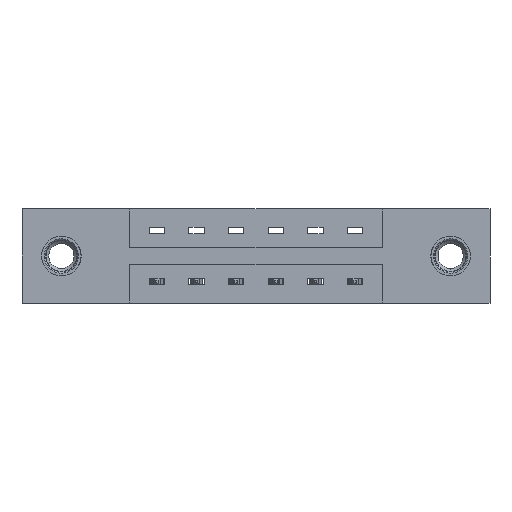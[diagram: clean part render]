
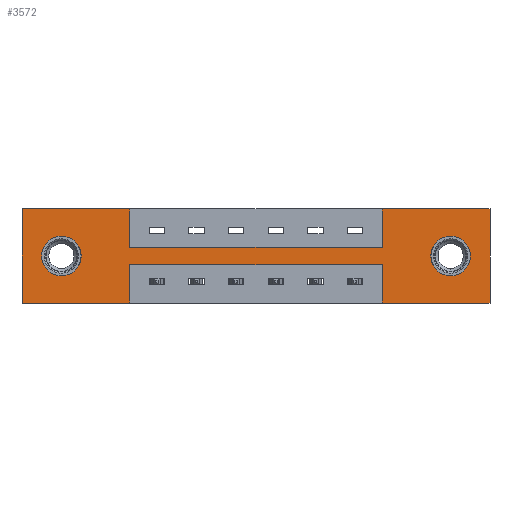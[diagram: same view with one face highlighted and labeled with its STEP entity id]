
A CAD part, front view. The second image highlights one B-rep face of the part: STEP entity #3572.
In plain terms, the highlighted planar face has unit normal (0, -1, 0).
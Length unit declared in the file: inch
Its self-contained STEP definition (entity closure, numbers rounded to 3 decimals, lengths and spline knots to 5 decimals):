
#15 = ORIENTED_EDGE ( 'NONE', *, *, #8971, .F. ) ;
#354 = LINE ( 'NONE', #3860, #2844 ) ;
#487 = VERTEX_POINT ( 'NONE', #9995 ) ;
#631 = EDGE_CURVE ( 'NONE', #6717, #3321, #6698, .T. ) ;
#673 = FACE_OUTER_BOUND ( 'NONE', #7245, .T. ) ;
#692 = LINE ( 'NONE', #9486, #9682 ) ;
#1028 = DIRECTION ( 'NONE',  ( 0., 0., -1. ) ) ;
#1061 = DIRECTION ( 'NONE',  ( 0., 1., 0. ) ) ;
#1080 = ORIENTED_EDGE ( 'NONE', *, *, #5668, .T. ) ;
#1142 = AXIS2_PLACEMENT_3D ( 'NONE', #9271, #4467, #6088 ) ;
#1146 = DIRECTION ( 'NONE',  ( 0., 0., 1. ) ) ;
#1313 = VECTOR ( 'NONE', #6585, 39.37008 ) ;
#1339 = CARTESIAN_POINT ( 'NONE',  ( 1.842, 0., -0.37 ) ) ;
#1387 = CARTESIAN_POINT ( 'NONE',  ( 0., 0., 0. ) ) ;
#1512 = VERTEX_POINT ( 'NONE', #10016 ) ;
#1695 = DIRECTION ( 'NONE',  ( -1., 0., 0. ) ) ;
#1712 = CARTESIAN_POINT ( 'NONE',  ( 1.842, 0., 0. ) ) ;
#1737 = CARTESIAN_POINT ( 'NONE',  ( 0.425, 0., -0.15 ) ) ;
#1751 = EDGE_CURVE ( 'NONE', #487, #3925, #10070, .T. ) ;
#1791 = VERTEX_POINT ( 'NONE', #8266 ) ;
#1977 = VERTEX_POINT ( 'NONE', #8176 ) ;
#1978 = EDGE_CURVE ( 'NONE', #3321, #1791, #3049, .T. ) ;
#2050 = EDGE_CURVE ( 'NONE', #9061, #5885, #9435, .T. ) ;
#2147 = AXIS2_PLACEMENT_3D ( 'NONE', #2590, #6578, #1028 ) ;
#2290 = DIRECTION ( 'NONE',  ( -1., 0., 0. ) ) ;
#2469 = EDGE_LOOP ( 'NONE', ( #5500, #4221 ) ) ;
#2579 = VERTEX_POINT ( 'NONE', #8426 ) ;
#2590 = CARTESIAN_POINT ( 'NONE',  ( 0., 0., -0.37 ) ) ;
#2623 = PLANE ( 'NONE',  #2147 ) ;
#2844 = VECTOR ( 'NONE', #2290, 39.37008 ) ;
#2908 = EDGE_CURVE ( 'NONE', #6254, #3053, #6924, .T. ) ;
#2949 = EDGE_CURVE ( 'NONE', #5885, #9061, #5907, .T. ) ;
#3049 = LINE ( 'NONE', #8140, #10303 ) ;
#3053 = VERTEX_POINT ( 'NONE', #1339 ) ;
#3117 = ORIENTED_EDGE ( 'NONE', *, *, #9688, .F. ) ;
#3219 = DIRECTION ( 'NONE',  ( 1., 0., 0. ) ) ;
#3321 = VERTEX_POINT ( 'NONE', #5565 ) ;
#3382 = CARTESIAN_POINT ( 'NONE',  ( 0.425, 0., -0.37 ) ) ;
#3572 = ADVANCED_FACE ( 'NONE', ( #8411, #6151, #673 ), #2623, .T. ) ;
#3645 = LINE ( 'NONE', #1737, #8407 ) ;
#3860 = CARTESIAN_POINT ( 'NONE',  ( 0.425, 0., -0.22 ) ) ;
#3925 = VERTEX_POINT ( 'NONE', #4367 ) ;
#3964 = LINE ( 'NONE', #4913, #5933 ) ;
#4069 = VERTEX_POINT ( 'NONE', #9632 ) ;
#4138 = CARTESIAN_POINT ( 'NONE',  ( 0., 0., -0.37 ) ) ;
#4189 = CIRCLE ( 'NONE', #4263, 0.078 ) ;
#4221 = ORIENTED_EDGE ( 'NONE', *, *, #2949, .T. ) ;
#4254 = DIRECTION ( 'NONE',  ( 0., 1., 0. ) ) ;
#4263 = AXIS2_PLACEMENT_3D ( 'NONE', #9015, #4254, #5082 ) ;
#4367 = CARTESIAN_POINT ( 'NONE',  ( 0.425, 0., -0.37 ) ) ;
#4467 = DIRECTION ( 'NONE',  ( 0., 1., 0. ) ) ;
#4578 = VECTOR ( 'NONE', #8750, 39.37008 ) ;
#4743 = EDGE_CURVE ( 'NONE', #7360, #487, #354, .T. ) ;
#4784 = VECTOR ( 'NONE', #7283, 39.37008 ) ;
#4875 = ORIENTED_EDGE ( 'NONE', *, *, #1751, .F. ) ;
#4887 = EDGE_CURVE ( 'NONE', #1512, #7360, #3964, .T. ) ;
#4913 = CARTESIAN_POINT ( 'NONE',  ( 1.417, 0., -0.37 ) ) ;
#4977 = DIRECTION ( 'NONE',  ( 0., 0., 1. ) ) ;
#5082 = DIRECTION ( 'NONE',  ( 0., 0., -1. ) ) ;
#5191 = ORIENTED_EDGE ( 'NONE', *, *, #631, .F. ) ;
#5242 = CARTESIAN_POINT ( 'NONE',  ( 0.155, 0., -0.107 ) ) ;
#5296 = ORIENTED_EDGE ( 'NONE', *, *, #4743, .F. ) ;
#5428 = CARTESIAN_POINT ( 'NONE',  ( 1.842, 0., 0. ) ) ;
#5453 = ORIENTED_EDGE ( 'NONE', *, *, #7942, .F. ) ;
#5500 = ORIENTED_EDGE ( 'NONE', *, *, #2050, .T. ) ;
#5565 = CARTESIAN_POINT ( 'NONE',  ( 0.425, 0., 0. ) ) ;
#5668 = EDGE_CURVE ( 'NONE', #4069, #9703, #7670, .T. ) ;
#5766 = CARTESIAN_POINT ( 'NONE',  ( 0., 0., 0. ) ) ;
#5828 = CARTESIAN_POINT ( 'NONE',  ( 0.155, 0., -0.185 ) ) ;
#5885 = VERTEX_POINT ( 'NONE', #10095 ) ;
#5907 = CIRCLE ( 'NONE', #8162, 0.078 ) ;
#5933 = VECTOR ( 'NONE', #4977, 39.37008 ) ;
#5948 = CARTESIAN_POINT ( 'NONE',  ( 0.155, 0., -0.185 ) ) ;
#5995 = EDGE_CURVE ( 'NONE', #1977, #6254, #692, .T. ) ;
#6088 = DIRECTION ( 'NONE',  ( 0., 0., -1. ) ) ;
#6122 = ORIENTED_EDGE ( 'NONE', *, *, #2908, .F. ) ;
#6151 = FACE_BOUND ( 'NONE', #2469, .T. ) ;
#6204 = CARTESIAN_POINT ( 'NONE',  ( 1.687, 0., -0.107 ) ) ;
#6254 = VERTEX_POINT ( 'NONE', #5428 ) ;
#6307 = VECTOR ( 'NONE', #1695, 39.37008 ) ;
#6378 = EDGE_CURVE ( 'NONE', #3053, #1512, #9427, .T. ) ;
#6511 = ORIENTED_EDGE ( 'NONE', *, *, #10229, .T. ) ;
#6578 = DIRECTION ( 'NONE',  ( 0., -1., 0. ) ) ;
#6585 = DIRECTION ( 'NONE',  ( 0., 0., -1. ) ) ;
#6698 = LINE ( 'NONE', #7125, #4578 ) ;
#6717 = VERTEX_POINT ( 'NONE', #5766 ) ;
#6924 = LINE ( 'NONE', #1712, #4784 ) ;
#6945 = AXIS2_PLACEMENT_3D ( 'NONE', #5948, #9094, #9063 ) ;
#6950 = CARTESIAN_POINT ( 'NONE',  ( 0., 0., -0.37 ) ) ;
#7111 = LINE ( 'NONE', #8177, #7736 ) ;
#7125 = CARTESIAN_POINT ( 'NONE',  ( 0., 0., 0. ) ) ;
#7216 = CARTESIAN_POINT ( 'NONE',  ( 0., 0., -0.37 ) ) ;
#7245 = EDGE_LOOP ( 'NONE', ( #4875, #5296, #8963, #9567, #6122, #7726, #15, #5453, #9311, #5191, #3117, #9150 ) ) ;
#7283 = DIRECTION ( 'NONE',  ( 0., 0., -1. ) ) ;
#7337 = DIRECTION ( 'NONE',  ( -1., 0., 0. ) ) ;
#7356 = VERTEX_POINT ( 'NONE', #7216 ) ;
#7360 = VERTEX_POINT ( 'NONE', #9666 ) ;
#7670 = CIRCLE ( 'NONE', #1142, 0.078 ) ;
#7726 = ORIENTED_EDGE ( 'NONE', *, *, #5995, .F. ) ;
#7736 = VECTOR ( 'NONE', #1146, 39.37008 ) ;
#7853 = EDGE_CURVE ( 'NONE', #3925, #7356, #10274, .T. ) ;
#7942 = EDGE_CURVE ( 'NONE', #1791, #2579, #3645, .T. ) ;
#7970 = EDGE_LOOP ( 'NONE', ( #6511, #1080 ) ) ;
#8140 = CARTESIAN_POINT ( 'NONE',  ( 0.425, 0., 0. ) ) ;
#8162 = AXIS2_PLACEMENT_3D ( 'NONE', #5828, #1061, #8291 ) ;
#8176 = CARTESIAN_POINT ( 'NONE',  ( 1.417, 0., 0. ) ) ;
#8177 = CARTESIAN_POINT ( 'NONE',  ( 1.417, 0., 0. ) ) ;
#8266 = CARTESIAN_POINT ( 'NONE',  ( 0.425, 0., -0.15 ) ) ;
#8291 = DIRECTION ( 'NONE',  ( 0., 0., 1. ) ) ;
#8407 = VECTOR ( 'NONE', #3219, 39.37008 ) ;
#8411 = FACE_BOUND ( 'NONE', #7970, .T. ) ;
#8426 = CARTESIAN_POINT ( 'NONE',  ( 1.417, 0., -0.15 ) ) ;
#8547 = DIRECTION ( 'NONE',  ( 0., 0., 1. ) ) ;
#8558 = DIRECTION ( 'NONE',  ( 1., 0., 0. ) ) ;
#8750 = DIRECTION ( 'NONE',  ( 1., 0., 0. ) ) ;
#8940 = DIRECTION ( 'NONE',  ( 0., 0., -1. ) ) ;
#8963 = ORIENTED_EDGE ( 'NONE', *, *, #4887, .F. ) ;
#8971 = EDGE_CURVE ( 'NONE', #2579, #1977, #7111, .T. ) ;
#9015 = CARTESIAN_POINT ( 'NONE',  ( 1.687, 0., -0.185 ) ) ;
#9061 = VERTEX_POINT ( 'NONE', #5242 ) ;
#9063 = DIRECTION ( 'NONE',  ( 0., 0., 1. ) ) ;
#9093 = VECTOR ( 'NONE', #8547, 39.37008 ) ;
#9094 = DIRECTION ( 'NONE',  ( 0., 1., 0. ) ) ;
#9150 = ORIENTED_EDGE ( 'NONE', *, *, #7853, .F. ) ;
#9271 = CARTESIAN_POINT ( 'NONE',  ( 1.687, 0., -0.185 ) ) ;
#9311 = ORIENTED_EDGE ( 'NONE', *, *, #1978, .F. ) ;
#9414 = VECTOR ( 'NONE', #7337, 39.37008 ) ;
#9427 = LINE ( 'NONE', #4138, #6307 ) ;
#9435 = CIRCLE ( 'NONE', #6945, 0.078 ) ;
#9486 = CARTESIAN_POINT ( 'NONE',  ( 0., 0., 0. ) ) ;
#9567 = ORIENTED_EDGE ( 'NONE', *, *, #6378, .F. ) ;
#9632 = CARTESIAN_POINT ( 'NONE',  ( 1.687, 0., -0.263 ) ) ;
#9666 = CARTESIAN_POINT ( 'NONE',  ( 1.417, 0., -0.22 ) ) ;
#9682 = VECTOR ( 'NONE', #8558, 39.37008 ) ;
#9688 = EDGE_CURVE ( 'NONE', #7356, #6717, #9733, .T. ) ;
#9703 = VERTEX_POINT ( 'NONE', #6204 ) ;
#9733 = LINE ( 'NONE', #1387, #9093 ) ;
#9995 = CARTESIAN_POINT ( 'NONE',  ( 0.425, 0., -0.22 ) ) ;
#10016 = CARTESIAN_POINT ( 'NONE',  ( 1.417, 0., -0.37 ) ) ;
#10070 = LINE ( 'NONE', #3382, #1313 ) ;
#10095 = CARTESIAN_POINT ( 'NONE',  ( 0.155, 0., -0.263 ) ) ;
#10229 = EDGE_CURVE ( 'NONE', #9703, #4069, #4189, .T. ) ;
#10274 = LINE ( 'NONE', #6950, #9414 ) ;
#10303 = VECTOR ( 'NONE', #8940, 39.37008 ) ;
